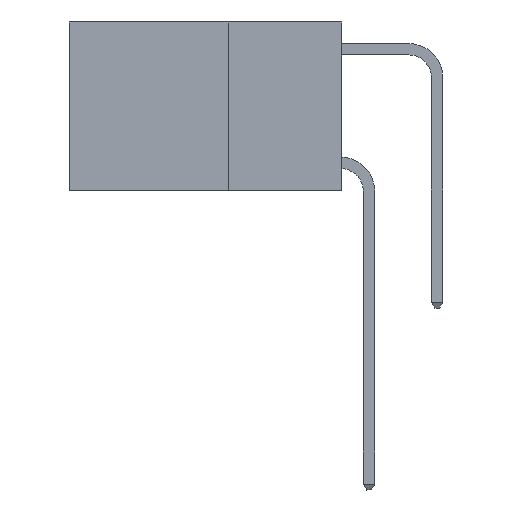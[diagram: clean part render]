
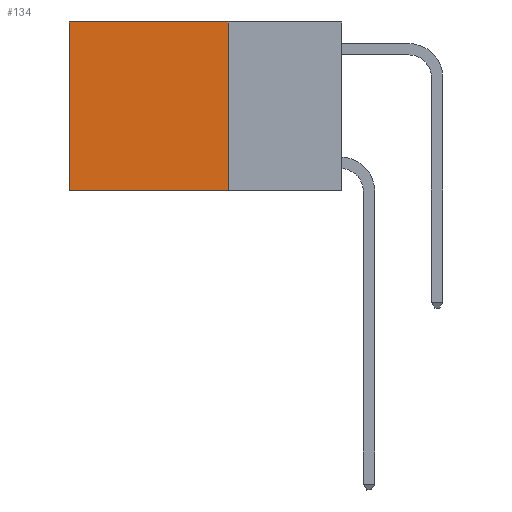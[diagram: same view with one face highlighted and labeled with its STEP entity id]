
A CAD part, left-side view. The second image highlights one B-rep face of the part: STEP entity #134.
In plain terms, the highlighted planar face has unit normal (-1, 0, 0).
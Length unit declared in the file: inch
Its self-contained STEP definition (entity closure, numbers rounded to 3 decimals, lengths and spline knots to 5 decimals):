
#134 = ADVANCED_FACE ( 'NONE', ( #13655 ), #10254, .F. ) ;
#479 = LINE ( 'NONE', #630, #9093 ) ;
#630 = CARTESIAN_POINT ( 'NONE',  ( 0.2625, 0.25, 0. ) ) ;
#746 = CARTESIAN_POINT ( 'NONE',  ( 0.2625, 0.25, 0. ) ) ;
#1151 = DIRECTION ( 'NONE',  ( 1., 0., 0. ) ) ;
#1205 = CARTESIAN_POINT ( 'NONE',  ( 0.2625, 0.6, -0.37 ) ) ;
#1369 = EDGE_LOOP ( 'NONE', ( #10070, #2422, #10250, #14537 ) ) ;
#1460 = EDGE_CURVE ( 'NONE', #1509, #12132, #11915, .T. ) ;
#1509 = VERTEX_POINT ( 'NONE', #15205 ) ;
#1530 = VECTOR ( 'NONE', #6345, 39.37008 ) ;
#1732 = AXIS2_PLACEMENT_3D ( 'NONE', #15140, #1151, #10311 ) ;
#1819 = CARTESIAN_POINT ( 'NONE',  ( 0.2625, 0.25, -0.37 ) ) ;
#1965 = VERTEX_POINT ( 'NONE', #6115 ) ;
#2079 = EDGE_CURVE ( 'NONE', #5547, #12132, #7133, .T. ) ;
#2422 = ORIENTED_EDGE ( 'NONE', *, *, #2079, .F. ) ;
#3746 = CARTESIAN_POINT ( 'NONE',  ( 0.2625, 0.6, 0. ) ) ;
#4836 = EDGE_CURVE ( 'NONE', #1965, #1509, #12078, .T. ) ;
#5547 = VERTEX_POINT ( 'NONE', #1819 ) ;
#6115 = CARTESIAN_POINT ( 'NONE',  ( 0.2625, 0.25, 0. ) ) ;
#6345 = DIRECTION ( 'NONE',  ( 0., 0., -1. ) ) ;
#6717 = VECTOR ( 'NONE', #16358, 39.37008 ) ;
#7133 = LINE ( 'NONE', #15138, #6717 ) ;
#7185 = EDGE_CURVE ( 'NONE', #1965, #5547, #479, .T. ) ;
#8293 = VECTOR ( 'NONE', #13567, 39.37008 ) ;
#8467 = DIRECTION ( 'NONE',  ( 0., 0., -1. ) ) ;
#9093 = VECTOR ( 'NONE', #8467, 39.37008 ) ;
#10070 = ORIENTED_EDGE ( 'NONE', *, *, #1460, .T. ) ;
#10250 = ORIENTED_EDGE ( 'NONE', *, *, #7185, .F. ) ;
#10254 = PLANE ( 'NONE',  #1732 ) ;
#10311 = DIRECTION ( 'NONE',  ( 0., 0., -1. ) ) ;
#11915 = LINE ( 'NONE', #3746, #1530 ) ;
#12078 = LINE ( 'NONE', #746, #8293 ) ;
#12132 = VERTEX_POINT ( 'NONE', #1205 ) ;
#13567 = DIRECTION ( 'NONE',  ( 0., 1., 0. ) ) ;
#13655 = FACE_OUTER_BOUND ( 'NONE', #1369, .T. ) ;
#14537 = ORIENTED_EDGE ( 'NONE', *, *, #4836, .T. ) ;
#15138 = CARTESIAN_POINT ( 'NONE',  ( 0.2625, 0.25, -0.37 ) ) ;
#15140 = CARTESIAN_POINT ( 'NONE',  ( 0.2625, 0.25, 0. ) ) ;
#15205 = CARTESIAN_POINT ( 'NONE',  ( 0.2625, 0.6, 0. ) ) ;
#16358 = DIRECTION ( 'NONE',  ( 0., 1., 0. ) ) ;
